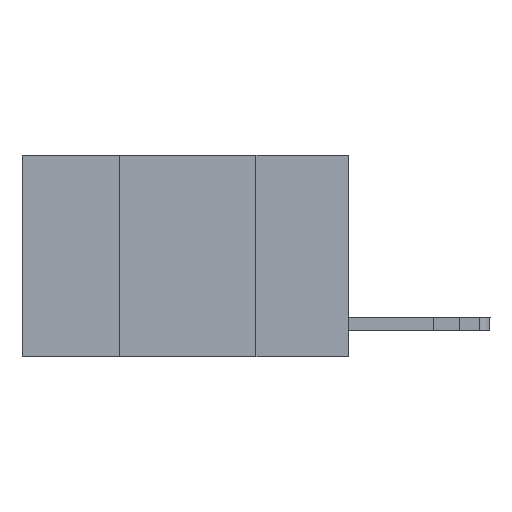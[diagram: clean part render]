
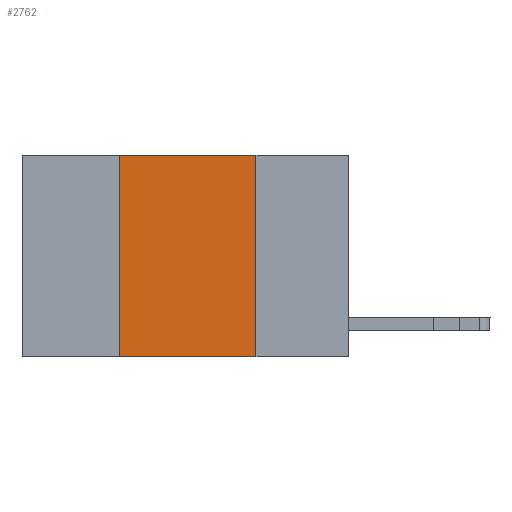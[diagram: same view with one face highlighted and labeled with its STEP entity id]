
A CAD part, left-side view. The second image highlights one B-rep face of the part: STEP entity #2762.
In plain terms, the highlighted planar face has unit normal (-1, 0, 0).
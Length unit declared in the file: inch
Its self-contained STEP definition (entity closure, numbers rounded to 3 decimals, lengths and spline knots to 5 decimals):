
#99 = ORIENTED_EDGE ( 'NONE', *, *, #8192, .T. ) ;
#711 = LINE ( 'NONE', #4029, #7050 ) ;
#897 = PLANE ( 'NONE',  #1360 ) ;
#1114 = CARTESIAN_POINT ( 'NONE',  ( 0., 0.6, 0. ) ) ;
#1360 = AXIS2_PLACEMENT_3D ( 'NONE', #1114, #2233, #6687 ) ;
#1788 = ORIENTED_EDGE ( 'NONE', *, *, #5556, .F. ) ;
#1846 = LINE ( 'NONE', #6158, #8344 ) ;
#1874 = LINE ( 'NONE', #11028, #13568 ) ;
#2233 = DIRECTION ( 'NONE',  ( 1., 0., 0. ) ) ;
#2762 = ADVANCED_FACE ( 'NONE', ( #13438 ), #897, .F. ) ;
#2912 = VECTOR ( 'NONE', #11771, 39.37008 ) ;
#3024 = EDGE_CURVE ( 'NONE', #7125, #6547, #1846, .T. ) ;
#3521 = CARTESIAN_POINT ( 'NONE',  ( 0., 0.42, 0. ) ) ;
#4029 = CARTESIAN_POINT ( 'NONE',  ( 0., 0.6, -0.37 ) ) ;
#5556 = EDGE_CURVE ( 'NONE', #6547, #13735, #1874, .T. ) ;
#6158 = CARTESIAN_POINT ( 'NONE',  ( 0., 0.42, 0. ) ) ;
#6547 = VERTEX_POINT ( 'NONE', #3521 ) ;
#6598 = VERTEX_POINT ( 'NONE', #9254 ) ;
#6687 = DIRECTION ( 'NONE',  ( 0., 0., -1. ) ) ;
#7050 = VECTOR ( 'NONE', #13997, 39.37008 ) ;
#7125 = VERTEX_POINT ( 'NONE', #12795 ) ;
#7324 = CARTESIAN_POINT ( 'NONE',  ( 0., 0.17, 0. ) ) ;
#7525 = ORIENTED_EDGE ( 'NONE', *, *, #12427, .F. ) ;
#8192 = EDGE_CURVE ( 'NONE', #7125, #6598, #711, .T. ) ;
#8344 = VECTOR ( 'NONE', #12783, 39.37008 ) ;
#8547 = LINE ( 'NONE', #7324, #2912 ) ;
#9254 = CARTESIAN_POINT ( 'NONE',  ( 0., 0.17, -0.37 ) ) ;
#10594 = CARTESIAN_POINT ( 'NONE',  ( 0., 0.17, 0. ) ) ;
#10809 = DIRECTION ( 'NONE',  ( 0., -1., 0. ) ) ;
#11028 = CARTESIAN_POINT ( 'NONE',  ( 0., 0.6, 0. ) ) ;
#11771 = DIRECTION ( 'NONE',  ( 0., 0., -1. ) ) ;
#12208 = ORIENTED_EDGE ( 'NONE', *, *, #3024, .F. ) ;
#12427 = EDGE_CURVE ( 'NONE', #13735, #6598, #8547, .T. ) ;
#12783 = DIRECTION ( 'NONE',  ( 0., 0., 1. ) ) ;
#12795 = CARTESIAN_POINT ( 'NONE',  ( 0., 0.42, -0.37 ) ) ;
#13245 = EDGE_LOOP ( 'NONE', ( #7525, #1788, #12208, #99 ) ) ;
#13438 = FACE_OUTER_BOUND ( 'NONE', #13245, .T. ) ;
#13568 = VECTOR ( 'NONE', #10809, 39.37008 ) ;
#13735 = VERTEX_POINT ( 'NONE', #10594 ) ;
#13997 = DIRECTION ( 'NONE',  ( 0., -1., 0. ) ) ;
